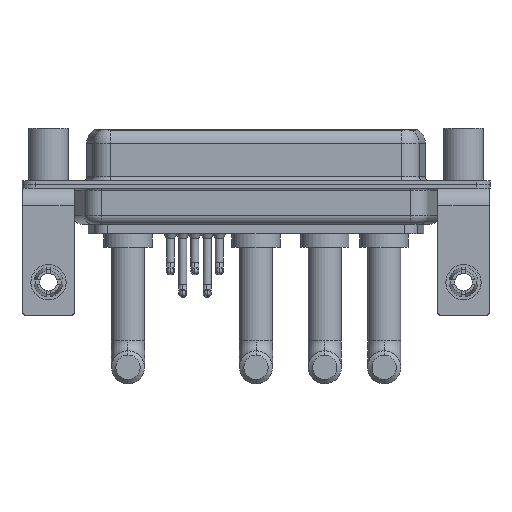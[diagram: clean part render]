
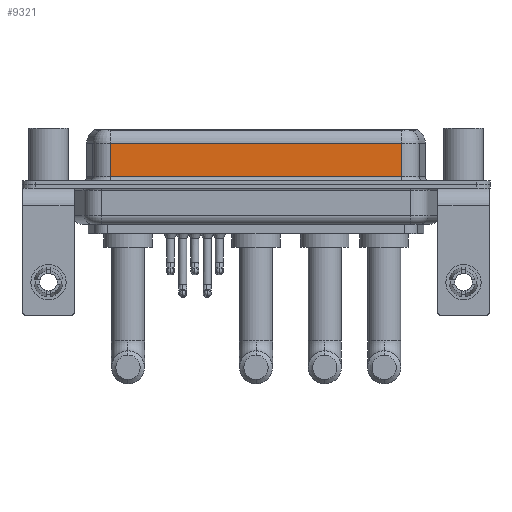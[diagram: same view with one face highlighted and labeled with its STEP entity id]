
A CAD part, front view. The second image highlights one B-rep face of the part: STEP entity #9321.
In plain terms, the highlighted planar face has unit normal (0, -1, 0).
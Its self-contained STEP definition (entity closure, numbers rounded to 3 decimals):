
#982 = LINE ( 'NONE', #5831, #5257 ) ;
#2420 = LINE ( 'NONE', #16882, #11446 ) ;
#3087 = VERTEX_POINT ( 'NONE', #9402 ) ;
#3377 = CARTESIAN_POINT ( 'NONE',  ( 40.037, -3.95, 0.9 ) ) ;
#3890 = VECTOR ( 'NONE', #14639, 1000. ) ;
#4049 = AXIS2_PLACEMENT_3D ( 'NONE', #8416, #11678, #18227 ) ;
#4267 = DIRECTION ( 'NONE',  ( 0., 0., -1. ) ) ;
#4852 = ORIENTED_EDGE ( 'NONE', *, *, #14326, .T. ) ;
#4957 = LINE ( 'NONE', #11362, #3890 ) ;
#5257 = VECTOR ( 'NONE', #4267, 1000. ) ;
#5831 = CARTESIAN_POINT ( 'NONE',  ( 7.013, -3.95, 6.4 ) ) ;
#6484 = ORIENTED_EDGE ( 'NONE', *, *, #13907, .T. ) ;
#7379 = ORIENTED_EDGE ( 'NONE', *, *, #10229, .F. ) ;
#7592 = VECTOR ( 'NONE', #13315, 1000. ) ;
#8033 = CARTESIAN_POINT ( 'NONE',  ( 40.037, -3.95, 4.65 ) ) ;
#8416 = CARTESIAN_POINT ( 'NONE',  ( 40.037, -3.95, 6.4 ) ) ;
#9321 = ADVANCED_FACE ( 'NONE', ( #10199 ), #10001, .F. ) ;
#9402 = CARTESIAN_POINT ( 'NONE',  ( 7.013, -3.95, 4.65 ) ) ;
#9463 = ORIENTED_EDGE ( 'NONE', *, *, #14612, .T. ) ;
#10001 = PLANE ( 'NONE',  #4049 ) ;
#10199 = FACE_OUTER_BOUND ( 'NONE', #18887, .T. ) ;
#10229 = EDGE_CURVE ( 'NONE', #11355, #15145, #2420, .T. ) ;
#11150 = CARTESIAN_POINT ( 'NONE',  ( 7.013, -3.95, 0.9 ) ) ;
#11355 = VERTEX_POINT ( 'NONE', #13150 ) ;
#11362 = CARTESIAN_POINT ( 'NONE',  ( 40.037, -3.95, 0.9 ) ) ;
#11446 = VECTOR ( 'NONE', #11815, 1000. ) ;
#11678 = DIRECTION ( 'NONE',  ( 0., 1., 0. ) ) ;
#11815 = DIRECTION ( 'NONE',  ( 0., 0., -1. ) ) ;
#13150 = CARTESIAN_POINT ( 'NONE',  ( 40.037, -3.95, 4.65 ) ) ;
#13315 = DIRECTION ( 'NONE',  ( -1., 0., 0. ) ) ;
#13907 = EDGE_CURVE ( 'NONE', #16920, #15145, #4957, .T. ) ;
#14326 = EDGE_CURVE ( 'NONE', #3087, #16920, #982, .T. ) ;
#14612 = EDGE_CURVE ( 'NONE', #11355, #3087, #19610, .T. ) ;
#14639 = DIRECTION ( 'NONE',  ( 1., 0., 0. ) ) ;
#15145 = VERTEX_POINT ( 'NONE', #3377 ) ;
#16882 = CARTESIAN_POINT ( 'NONE',  ( 40.037, -3.95, 6.4 ) ) ;
#16920 = VERTEX_POINT ( 'NONE', #11150 ) ;
#18227 = DIRECTION ( 'NONE',  ( 0., 0., 1. ) ) ;
#18887 = EDGE_LOOP ( 'NONE', ( #7379, #9463, #4852, #6484 ) ) ;
#19610 = LINE ( 'NONE', #8033, #7592 ) ;
